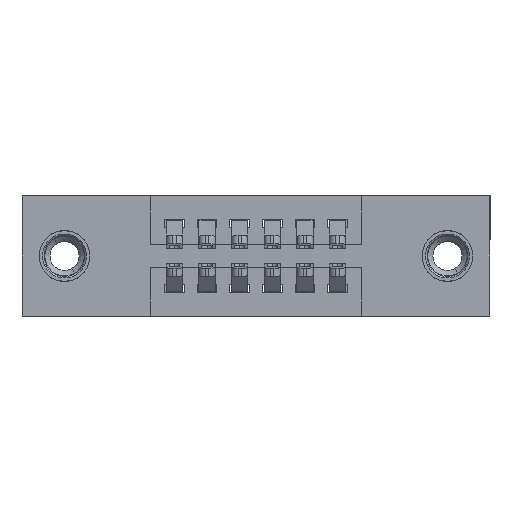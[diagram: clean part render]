
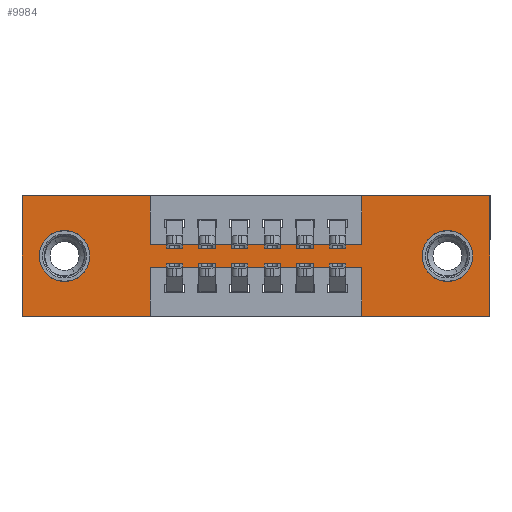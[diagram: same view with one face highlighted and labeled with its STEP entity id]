
A CAD part, front view. The second image highlights one B-rep face of the part: STEP entity #9984.
In plain terms, the highlighted planar face has unit normal (0, -1, 0).
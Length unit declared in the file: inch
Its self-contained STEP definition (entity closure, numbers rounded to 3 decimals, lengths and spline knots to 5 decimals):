
#51 = CARTESIAN_POINT ( 'NONE',  ( 0.3925, 0., -0.22 ) ) ;
#152 = VECTOR ( 'NONE', #4513, 39.37008 ) ;
#240 = CARTESIAN_POINT ( 'NONE',  ( 0.13, 0., -0.107 ) ) ;
#271 = ORIENTED_EDGE ( 'NONE', *, *, #14657, .F. ) ;
#356 = LINE ( 'NONE', #3499, #9174 ) ;
#398 = EDGE_LOOP ( 'NONE', ( #1979, #1316 ) ) ;
#437 = ORIENTED_EDGE ( 'NONE', *, *, #6683, .F. ) ;
#460 = CARTESIAN_POINT ( 'NONE',  ( 0., 0., -0.37 ) ) ;
#520 = CARTESIAN_POINT ( 'NONE',  ( 0., 0., -0.37 ) ) ;
#787 = EDGE_CURVE ( 'NONE', #7752, #1385, #5336, .T. ) ;
#945 = FACE_OUTER_BOUND ( 'NONE', #11900, .T. ) ;
#1188 = DIRECTION ( 'NONE',  ( 0., 0., -1. ) ) ;
#1316 = ORIENTED_EDGE ( 'NONE', *, *, #13427, .T. ) ;
#1385 = VERTEX_POINT ( 'NONE', #3876 ) ;
#1590 = CARTESIAN_POINT ( 'NONE',  ( 1.305, 0., -0.263 ) ) ;
#1614 = CARTESIAN_POINT ( 'NONE',  ( 1.0425, 0., -0.37 ) ) ;
#1637 = DIRECTION ( 'NONE',  ( 0., 0., -1. ) ) ;
#1651 = DIRECTION ( 'NONE',  ( 0., 1., 0. ) ) ;
#1709 = CARTESIAN_POINT ( 'NONE',  ( 1.305, 0., -0.185 ) ) ;
#1801 = ORIENTED_EDGE ( 'NONE', *, *, #13895, .F. ) ;
#1872 = DIRECTION ( 'NONE',  ( 0., 1., 0. ) ) ;
#1979 = ORIENTED_EDGE ( 'NONE', *, *, #3960, .T. ) ;
#2024 = LINE ( 'NONE', #13516, #13890 ) ;
#3043 = ORIENTED_EDGE ( 'NONE', *, *, #14149, .F. ) ;
#3135 = VECTOR ( 'NONE', #13614, 39.37008 ) ;
#3274 = EDGE_LOOP ( 'NONE', ( #4857, #12456 ) ) ;
#3318 = LINE ( 'NONE', #4109, #8919 ) ;
#3380 = VECTOR ( 'NONE', #8569, 39.37008 ) ;
#3393 = VECTOR ( 'NONE', #5206, 39.37008 ) ;
#3431 = ORIENTED_EDGE ( 'NONE', *, *, #10458, .F. ) ;
#3499 = CARTESIAN_POINT ( 'NONE',  ( 1.435, 0., 0. ) ) ;
#3590 = CARTESIAN_POINT ( 'NONE',  ( 1.0425, 0., -0.15 ) ) ;
#3772 = LINE ( 'NONE', #10047, #152 ) ;
#3792 = EDGE_CURVE ( 'NONE', #12862, #5573, #3318, .T. ) ;
#3876 = CARTESIAN_POINT ( 'NONE',  ( 1.435, 0., 0. ) ) ;
#3960 = EDGE_CURVE ( 'NONE', #11127, #4201, #13005, .T. ) ;
#4035 = DIRECTION ( 'NONE',  ( 0., 0., -1. ) ) ;
#4084 = CARTESIAN_POINT ( 'NONE',  ( 0., 0., 0. ) ) ;
#4109 = CARTESIAN_POINT ( 'NONE',  ( 0.3925, 0., -0.37 ) ) ;
#4138 = ORIENTED_EDGE ( 'NONE', *, *, #3792, .F. ) ;
#4201 = VERTEX_POINT ( 'NONE', #1590 ) ;
#4513 = DIRECTION ( 'NONE',  ( 0., 0., 1. ) ) ;
#4584 = CARTESIAN_POINT ( 'NONE',  ( 0., 0., 0. ) ) ;
#4845 = VERTEX_POINT ( 'NONE', #9482 ) ;
#4857 = ORIENTED_EDGE ( 'NONE', *, *, #6848, .T. ) ;
#4874 = CARTESIAN_POINT ( 'NONE',  ( 1.0425, 0., -0.22 ) ) ;
#5008 = CIRCLE ( 'NONE', #13187, 0.078 ) ;
#5171 = CARTESIAN_POINT ( 'NONE',  ( 0.13, 0., -0.185 ) ) ;
#5205 = EDGE_CURVE ( 'NONE', #9267, #12862, #13899, .T. ) ;
#5206 = DIRECTION ( 'NONE',  ( 0., 0., 1. ) ) ;
#5336 = LINE ( 'NONE', #9869, #10544 ) ;
#5461 = CARTESIAN_POINT ( 'NONE',  ( 0.3925, 0., 0. ) ) ;
#5573 = VERTEX_POINT ( 'NONE', #6719 ) ;
#5631 = CARTESIAN_POINT ( 'NONE',  ( 1.0425, 0., 0. ) ) ;
#5673 = VERTEX_POINT ( 'NONE', #14553 ) ;
#5693 = EDGE_CURVE ( 'NONE', #10426, #11307, #2024, .T. ) ;
#6105 = LINE ( 'NONE', #12504, #3135 ) ;
#6277 = DIRECTION ( 'NONE',  ( 0., 0., 1. ) ) ;
#6292 = DIRECTION ( 'NONE',  ( -1., 0., 0. ) ) ;
#6304 = DIRECTION ( 'NONE',  ( 0., -1., 0. ) ) ;
#6683 = EDGE_CURVE ( 'NONE', #9066, #13791, #6105, .T. ) ;
#6708 = FACE_BOUND ( 'NONE', #398, .T. ) ;
#6719 = CARTESIAN_POINT ( 'NONE',  ( 0.3925, 0., -0.37 ) ) ;
#6763 = VECTOR ( 'NONE', #8456, 39.37008 ) ;
#6848 = EDGE_CURVE ( 'NONE', #11481, #4845, #7315, .T. ) ;
#6901 = DIRECTION ( 'NONE',  ( 1., 0., 0. ) ) ;
#6915 = CARTESIAN_POINT ( 'NONE',  ( 0.3925, 0., -0.22 ) ) ;
#7315 = CIRCLE ( 'NONE', #13594, 0.078 ) ;
#7409 = CARTESIAN_POINT ( 'NONE',  ( 0., 0., -0.37 ) ) ;
#7652 = AXIS2_PLACEMENT_3D ( 'NONE', #8684, #1872, #9797 ) ;
#7709 = VECTOR ( 'NONE', #11429, 39.37008 ) ;
#7752 = VERTEX_POINT ( 'NONE', #5631 ) ;
#7813 = VERTEX_POINT ( 'NONE', #13445 ) ;
#7843 = ORIENTED_EDGE ( 'NONE', *, *, #8107, .F. ) ;
#8048 = DIRECTION ( 'NONE',  ( 0., 1., 0. ) ) ;
#8107 = EDGE_CURVE ( 'NONE', #5673, #9267, #12286, .T. ) ;
#8456 = DIRECTION ( 'NONE',  ( 0., 0., 1. ) ) ;
#8534 = CIRCLE ( 'NONE', #7652, 0.078 ) ;
#8569 = DIRECTION ( 'NONE',  ( -1., 0., 0. ) ) ;
#8684 = CARTESIAN_POINT ( 'NONE',  ( 0.13, 0., -0.185 ) ) ;
#8919 = VECTOR ( 'NONE', #4035, 39.37008 ) ;
#8997 = DIRECTION ( 'NONE',  ( 0., 0., -1. ) ) ;
#9066 = VERTEX_POINT ( 'NONE', #4584 ) ;
#9174 = VECTOR ( 'NONE', #11217, 39.37008 ) ;
#9267 = VERTEX_POINT ( 'NONE', #4874 ) ;
#9337 = ORIENTED_EDGE ( 'NONE', *, *, #14424, .F. ) ;
#9345 = LINE ( 'NONE', #4084, #3393 ) ;
#9482 = CARTESIAN_POINT ( 'NONE',  ( 0.13, 0., -0.263 ) ) ;
#9612 = AXIS2_PLACEMENT_3D ( 'NONE', #460, #6304, #14017 ) ;
#9683 = FACE_BOUND ( 'NONE', #3274, .T. ) ;
#9797 = DIRECTION ( 'NONE',  ( 0., 0., 1. ) ) ;
#9837 = CARTESIAN_POINT ( 'NONE',  ( 1.305, 0., -0.107 ) ) ;
#9859 = LINE ( 'NONE', #7409, #12405 ) ;
#9869 = CARTESIAN_POINT ( 'NONE',  ( 0., 0., 0. ) ) ;
#9984 = ADVANCED_FACE ( 'NONE', ( #6708, #9683, #945 ), #11829, .T. ) ;
#9991 = DIRECTION ( 'NONE',  ( 1., 0., 0. ) ) ;
#10047 = CARTESIAN_POINT ( 'NONE',  ( 1.0425, 0., 0. ) ) ;
#10242 = EDGE_CURVE ( 'NONE', #11307, #7752, #3772, .T. ) ;
#10426 = VERTEX_POINT ( 'NONE', #13906 ) ;
#10458 = EDGE_CURVE ( 'NONE', #5573, #13021, #9859, .T. ) ;
#10544 = VECTOR ( 'NONE', #9991, 39.37008 ) ;
#10825 = ORIENTED_EDGE ( 'NONE', *, *, #5693, .F. ) ;
#11127 = VERTEX_POINT ( 'NONE', #9837 ) ;
#11217 = DIRECTION ( 'NONE',  ( 0., 0., -1. ) ) ;
#11307 = VERTEX_POINT ( 'NONE', #3590 ) ;
#11429 = DIRECTION ( 'NONE',  ( -1., 0., 0. ) ) ;
#11481 = VERTEX_POINT ( 'NONE', #240 ) ;
#11523 = ORIENTED_EDGE ( 'NONE', *, *, #787, .F. ) ;
#11556 = LINE ( 'NONE', #520, #3380 ) ;
#11730 = VECTOR ( 'NONE', #8997, 39.37008 ) ;
#11829 = PLANE ( 'NONE',  #9612 ) ;
#11900 = EDGE_LOOP ( 'NONE', ( #4138, #12949, #7843, #271, #1801, #11523, #13808, #10825, #9337, #437, #3043, #3431 ) ) ;
#12144 = EDGE_CURVE ( 'NONE', #4845, #11481, #8534, .T. ) ;
#12286 = LINE ( 'NONE', #1614, #6763 ) ;
#12352 = AXIS2_PLACEMENT_3D ( 'NONE', #1709, #1651, #1637 ) ;
#12405 = VECTOR ( 'NONE', #6292, 39.37008 ) ;
#12456 = ORIENTED_EDGE ( 'NONE', *, *, #12144, .T. ) ;
#12504 = CARTESIAN_POINT ( 'NONE',  ( 0., 0., 0. ) ) ;
#12861 = DIRECTION ( 'NONE',  ( 0., 1., 0. ) ) ;
#12862 = VERTEX_POINT ( 'NONE', #51 ) ;
#12949 = ORIENTED_EDGE ( 'NONE', *, *, #5205, .F. ) ;
#13005 = CIRCLE ( 'NONE', #12352, 0.078 ) ;
#13021 = VERTEX_POINT ( 'NONE', #13860 ) ;
#13187 = AXIS2_PLACEMENT_3D ( 'NONE', #14611, #8048, #1188 ) ;
#13352 = CARTESIAN_POINT ( 'NONE',  ( 0.3925, 0., 0. ) ) ;
#13427 = EDGE_CURVE ( 'NONE', #4201, #11127, #5008, .T. ) ;
#13445 = CARTESIAN_POINT ( 'NONE',  ( 1.435, 0., -0.37 ) ) ;
#13516 = CARTESIAN_POINT ( 'NONE',  ( 0.3925, 0., -0.15 ) ) ;
#13594 = AXIS2_PLACEMENT_3D ( 'NONE', #5171, #12861, #6277 ) ;
#13614 = DIRECTION ( 'NONE',  ( 1., 0., 0. ) ) ;
#13791 = VERTEX_POINT ( 'NONE', #5461 ) ;
#13808 = ORIENTED_EDGE ( 'NONE', *, *, #10242, .F. ) ;
#13860 = CARTESIAN_POINT ( 'NONE',  ( 0., 0., -0.37 ) ) ;
#13890 = VECTOR ( 'NONE', #6901, 39.37008 ) ;
#13895 = EDGE_CURVE ( 'NONE', #1385, #7813, #356, .T. ) ;
#13899 = LINE ( 'NONE', #6915, #7709 ) ;
#13906 = CARTESIAN_POINT ( 'NONE',  ( 0.3925, 0., -0.15 ) ) ;
#14017 = DIRECTION ( 'NONE',  ( 0., 0., -1. ) ) ;
#14149 = EDGE_CURVE ( 'NONE', #13021, #9066, #9345, .T. ) ;
#14424 = EDGE_CURVE ( 'NONE', #13791, #10426, #14622, .T. ) ;
#14553 = CARTESIAN_POINT ( 'NONE',  ( 1.0425, 0., -0.37 ) ) ;
#14611 = CARTESIAN_POINT ( 'NONE',  ( 1.305, 0., -0.185 ) ) ;
#14622 = LINE ( 'NONE', #13352, #11730 ) ;
#14657 = EDGE_CURVE ( 'NONE', #7813, #5673, #11556, .T. ) ;
